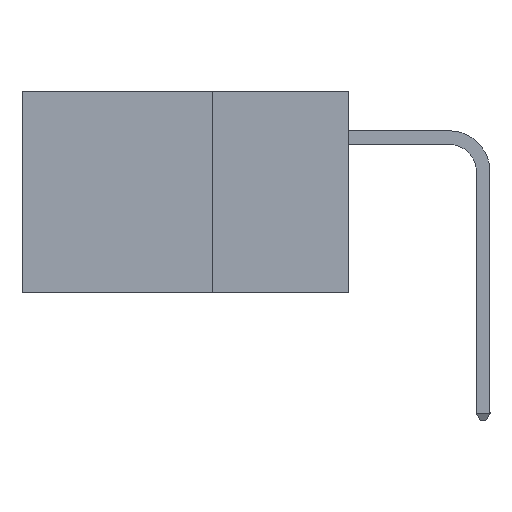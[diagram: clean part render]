
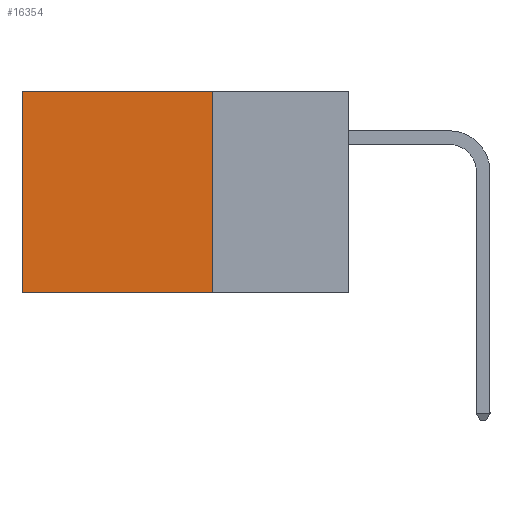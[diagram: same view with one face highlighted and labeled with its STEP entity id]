
A CAD part, left-side view. The second image highlights one B-rep face of the part: STEP entity #16354.
In plain terms, the highlighted planar face has unit normal (-1, 0, 0).
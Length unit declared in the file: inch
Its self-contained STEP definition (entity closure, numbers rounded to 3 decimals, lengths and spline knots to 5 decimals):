
#410 = LINE ( 'NONE', #24032, #38179 ) ;
#1446 = CARTESIAN_POINT ( 'NONE',  ( 0.2875, 0.25, 0. ) ) ;
#3483 = VERTEX_POINT ( 'NONE', #5817 ) ;
#3657 = CARTESIAN_POINT ( 'NONE',  ( 0.2875, 0.25, -0.37 ) ) ;
#3793 = EDGE_CURVE ( 'NONE', #33159, #29259, #26230, .T. ) ;
#3813 = VERTEX_POINT ( 'NONE', #16599 ) ;
#5817 = CARTESIAN_POINT ( 'NONE',  ( 0.2875, 0.25, 0. ) ) ;
#7559 = DIRECTION ( 'NONE',  ( 0., 0., -1. ) ) ;
#8502 = EDGE_CURVE ( 'NONE', #3483, #33159, #410, .T. ) ;
#9058 = ORIENTED_EDGE ( 'NONE', *, *, #24051, .F. ) ;
#10502 = CARTESIAN_POINT ( 'NONE',  ( 0.2875, 0.6, 0. ) ) ;
#13462 = ORIENTED_EDGE ( 'NONE', *, *, #3793, .T. ) ;
#13719 = AXIS2_PLACEMENT_3D ( 'NONE', #1446, #26247, #7559 ) ;
#15673 = DIRECTION ( 'NONE',  ( 0., 1., 0. ) ) ;
#15853 = LINE ( 'NONE', #3657, #16053 ) ;
#16053 = VECTOR ( 'NONE', #15673, 39.37008 ) ;
#16060 = LINE ( 'NONE', #37318, #16065 ) ;
#16065 = VECTOR ( 'NONE', #34166, 39.37008 ) ;
#16354 = ADVANCED_FACE ( 'NONE', ( #34544 ), #28420, .F. ) ;
#16599 = CARTESIAN_POINT ( 'NONE',  ( 0.2875, 0.25, -0.37 ) ) ;
#17924 = DIRECTION ( 'NONE',  ( 0., 1., 0. ) ) ;
#19946 = CARTESIAN_POINT ( 'NONE',  ( 0.2875, 0.6, 0. ) ) ;
#20282 = CARTESIAN_POINT ( 'NONE',  ( 0.2875, 0.6, -0.37 ) ) ;
#22171 = ORIENTED_EDGE ( 'NONE', *, *, #32749, .F. ) ;
#23597 = VECTOR ( 'NONE', #37678, 39.37008 ) ;
#24032 = CARTESIAN_POINT ( 'NONE',  ( 0.2875, 0.25, 0. ) ) ;
#24051 = EDGE_CURVE ( 'NONE', #3813, #29259, #15853, .T. ) ;
#26230 = LINE ( 'NONE', #19946, #23597 ) ;
#26247 = DIRECTION ( 'NONE',  ( 1., 0., 0. ) ) ;
#28420 = PLANE ( 'NONE',  #13719 ) ;
#29259 = VERTEX_POINT ( 'NONE', #20282 ) ;
#32749 = EDGE_CURVE ( 'NONE', #3483, #3813, #16060, .T. ) ;
#33159 = VERTEX_POINT ( 'NONE', #10502 ) ;
#34166 = DIRECTION ( 'NONE',  ( 0., 0., -1. ) ) ;
#34544 = FACE_OUTER_BOUND ( 'NONE', #38841, .T. ) ;
#34783 = ORIENTED_EDGE ( 'NONE', *, *, #8502, .T. ) ;
#37318 = CARTESIAN_POINT ( 'NONE',  ( 0.2875, 0.25, 0. ) ) ;
#37678 = DIRECTION ( 'NONE',  ( 0., 0., -1. ) ) ;
#38179 = VECTOR ( 'NONE', #17924, 39.37008 ) ;
#38841 = EDGE_LOOP ( 'NONE', ( #13462, #9058, #22171, #34783 ) ) ;
